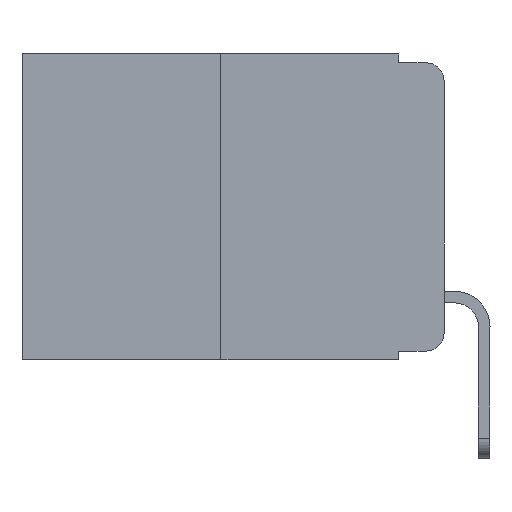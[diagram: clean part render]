
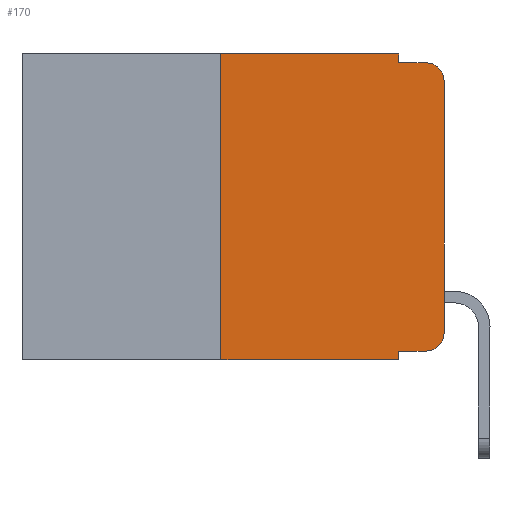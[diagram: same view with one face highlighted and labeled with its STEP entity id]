
A CAD part, left-side view. The second image highlights one B-rep face of the part: STEP entity #170.
In plain terms, the highlighted planar face has unit normal (-1, 0, 0).
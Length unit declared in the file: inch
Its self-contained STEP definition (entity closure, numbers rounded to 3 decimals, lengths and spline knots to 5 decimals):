
#170 = ADVANCED_FACE ( 'NONE', ( #5471 ), #10010, .F. ) ;
#393 = VECTOR ( 'NONE', #7949, 39.37008 ) ;
#420 = VERTEX_POINT ( 'NONE', #8793 ) ;
#549 = EDGE_CURVE ( 'NONE', #806, #10150, #2171, .T. ) ;
#806 = VERTEX_POINT ( 'NONE', #9032 ) ;
#813 = ORIENTED_EDGE ( 'NONE', *, *, #549, .F. ) ;
#989 = ORIENTED_EDGE ( 'NONE', *, *, #5341, .F. ) ;
#1258 = DIRECTION ( 'NONE',  ( 0., -1., 0. ) ) ;
#1483 = VERTEX_POINT ( 'NONE', #8061 ) ;
#1526 = CARTESIAN_POINT ( 'NONE',  ( 0., 0.473, 0. ) ) ;
#1554 = VERTEX_POINT ( 'NONE', #11098 ) ;
#1736 = VERTEX_POINT ( 'NONE', #4970 ) ;
#1908 = EDGE_CURVE ( 'NONE', #1736, #4803, #8378, .T. ) ;
#1918 = ORIENTED_EDGE ( 'NONE', *, *, #9752, .T. ) ;
#2171 = LINE ( 'NONE', #1526, #11847 ) ;
#2274 = DIRECTION ( 'NONE',  ( 0., 0., 1. ) ) ;
#2780 = CARTESIAN_POINT ( 'NONE',  ( 0., 0.051, -0.343 ) ) ;
#3002 = VECTOR ( 'NONE', #8241, 39.37008 ) ;
#3432 = LINE ( 'NONE', #7098, #393 ) ;
#3465 = VECTOR ( 'NONE', #6410, 39.37008 ) ;
#3928 = CIRCLE ( 'NONE', #10419, 0.02 ) ;
#4029 = DIRECTION ( 'NONE',  ( 0., 0., 1. ) ) ;
#4247 = VECTOR ( 'NONE', #6924, 39.37008 ) ;
#4275 = ORIENTED_EDGE ( 'NONE', *, *, #1908, .T. ) ;
#4407 = LINE ( 'NONE', #11083, #7219 ) ;
#4427 = LINE ( 'NONE', #5448, #3465 ) ;
#4504 = AXIS2_PLACEMENT_3D ( 'NONE', #9893, #9906, #8369 ) ;
#4596 = CARTESIAN_POINT ( 'NONE',  ( 0., 0.051, 0. ) ) ;
#4760 = VERTEX_POINT ( 'NONE', #8791 ) ;
#4803 = VERTEX_POINT ( 'NONE', #12151 ) ;
#4970 = CARTESIAN_POINT ( 'NONE',  ( 0., 0., -0.03 ) ) ;
#5014 = ORIENTED_EDGE ( 'NONE', *, *, #7582, .F. ) ;
#5079 = VECTOR ( 'NONE', #4029, 39.37008 ) ;
#5341 = EDGE_CURVE ( 'NONE', #1554, #4803, #6771, .T. ) ;
#5448 = CARTESIAN_POINT ( 'NONE',  ( 0., 0.473, -0.343 ) ) ;
#5471 = FACE_OUTER_BOUND ( 'NONE', #10604, .T. ) ;
#5550 = DIRECTION ( 'NONE',  ( -1., 0., 0. ) ) ;
#5744 = DIRECTION ( 'NONE',  ( 0., -1., 0. ) ) ;
#5990 = VECTOR ( 'NONE', #2274, 39.37008 ) ;
#6086 = VERTEX_POINT ( 'NONE', #2780 ) ;
#6302 = LINE ( 'NONE', #10799, #5990 ) ;
#6318 = CARTESIAN_POINT ( 'NONE',  ( 0., 0.02, -0.03 ) ) ;
#6410 = DIRECTION ( 'NONE',  ( 0., -1., 0. ) ) ;
#6771 = LINE ( 'NONE', #9542, #4247 ) ;
#6873 = CARTESIAN_POINT ( 'NONE',  ( 0., 0.051, 0. ) ) ;
#6924 = DIRECTION ( 'NONE',  ( 0., -1., 0. ) ) ;
#7098 = CARTESIAN_POINT ( 'NONE',  ( 0., 0.051, 0. ) ) ;
#7155 = ORIENTED_EDGE ( 'NONE', *, *, #8200, .T. ) ;
#7219 = VECTOR ( 'NONE', #5744, 39.37008 ) ;
#7269 = LINE ( 'NONE', #10422, #5079 ) ;
#7471 = CARTESIAN_POINT ( 'NONE',  ( 0., 0.051, -0.333 ) ) ;
#7518 = EDGE_CURVE ( 'NONE', #4760, #806, #6302, .T. ) ;
#7582 = EDGE_CURVE ( 'NONE', #10150, #1554, #10157, .T. ) ;
#7936 = VERTEX_POINT ( 'NONE', #7471 ) ;
#7949 = DIRECTION ( 'NONE',  ( 0., 0., -1. ) ) ;
#8061 = CARTESIAN_POINT ( 'NONE',  ( 0., 0.02, -0.333 ) ) ;
#8200 = EDGE_CURVE ( 'NONE', #420, #1736, #7269, .T. ) ;
#8241 = DIRECTION ( 'NONE',  ( 0., 0., -1. ) ) ;
#8369 = DIRECTION ( 'NONE',  ( 0., 0., -1. ) ) ;
#8378 = CIRCLE ( 'NONE', #10279, 0.02 ) ;
#8791 = CARTESIAN_POINT ( 'NONE',  ( 0., 0.25, -0.343 ) ) ;
#8793 = CARTESIAN_POINT ( 'NONE',  ( 0., 0., -0.313 ) ) ;
#9032 = CARTESIAN_POINT ( 'NONE',  ( 0., 0.25, 0. ) ) ;
#9542 = CARTESIAN_POINT ( 'NONE',  ( 0., 0.051, -0.01 ) ) ;
#9579 = ORIENTED_EDGE ( 'NONE', *, *, #10611, .T. ) ;
#9752 = EDGE_CURVE ( 'NONE', #4760, #6086, #4427, .T. ) ;
#9893 = CARTESIAN_POINT ( 'NONE',  ( 0., 0.473, 0. ) ) ;
#9906 = DIRECTION ( 'NONE',  ( 1., 0., 0. ) ) ;
#10010 = PLANE ( 'NONE',  #4504 ) ;
#10056 = DIRECTION ( 'NONE',  ( -1., 0., 0. ) ) ;
#10150 = VERTEX_POINT ( 'NONE', #6873 ) ;
#10152 = ORIENTED_EDGE ( 'NONE', *, *, #10767, .T. ) ;
#10157 = LINE ( 'NONE', #4596, #3002 ) ;
#10197 = DIRECTION ( 'NONE',  ( 0., 0., -1. ) ) ;
#10279 = AXIS2_PLACEMENT_3D ( 'NONE', #6318, #10056, #10197 ) ;
#10419 = AXIS2_PLACEMENT_3D ( 'NONE', #10898, #5550, #11769 ) ;
#10422 = CARTESIAN_POINT ( 'NONE',  ( 0., 0., 0. ) ) ;
#10591 = ORIENTED_EDGE ( 'NONE', *, *, #7518, .F. ) ;
#10604 = EDGE_LOOP ( 'NONE', ( #7155, #4275, #989, #5014, #813, #10591, #1918, #11274, #10152, #9579 ) ) ;
#10611 = EDGE_CURVE ( 'NONE', #1483, #420, #3928, .T. ) ;
#10767 = EDGE_CURVE ( 'NONE', #7936, #1483, #4407, .T. ) ;
#10799 = CARTESIAN_POINT ( 'NONE',  ( 0., 0.25, 0. ) ) ;
#10827 = EDGE_CURVE ( 'NONE', #7936, #6086, #3432, .T. ) ;
#10898 = CARTESIAN_POINT ( 'NONE',  ( 0., 0.02, -0.313 ) ) ;
#11083 = CARTESIAN_POINT ( 'NONE',  ( 0., 0.051, -0.333 ) ) ;
#11098 = CARTESIAN_POINT ( 'NONE',  ( 0., 0.051, -0.01 ) ) ;
#11274 = ORIENTED_EDGE ( 'NONE', *, *, #10827, .F. ) ;
#11769 = DIRECTION ( 'NONE',  ( 0., 0., -1. ) ) ;
#11847 = VECTOR ( 'NONE', #1258, 39.37008 ) ;
#12151 = CARTESIAN_POINT ( 'NONE',  ( 0., 0.02, -0.01 ) ) ;
